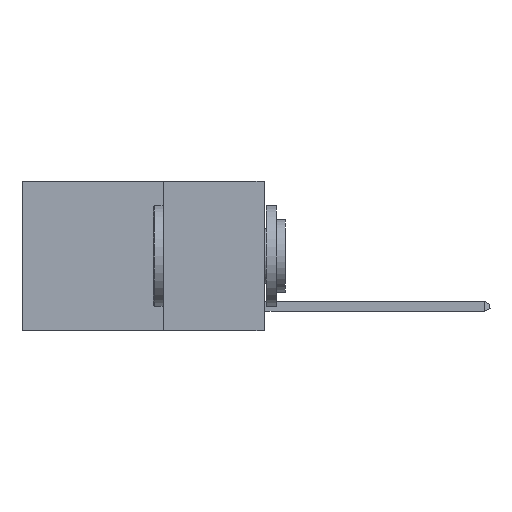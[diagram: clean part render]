
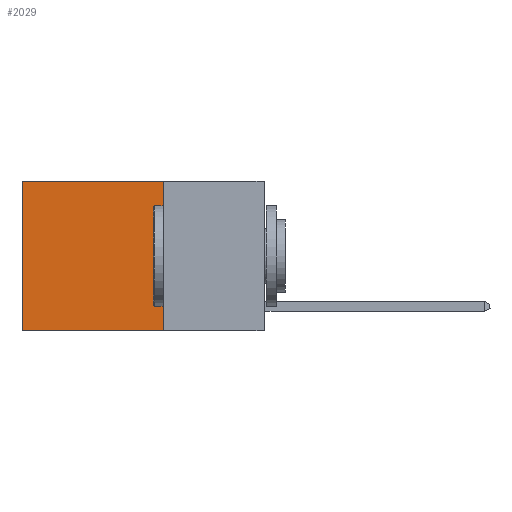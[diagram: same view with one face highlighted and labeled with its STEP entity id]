
A CAD part, left-side view. The second image highlights one B-rep face of the part: STEP entity #2029.
In plain terms, the highlighted planar face has unit normal (-1, 0, 0).
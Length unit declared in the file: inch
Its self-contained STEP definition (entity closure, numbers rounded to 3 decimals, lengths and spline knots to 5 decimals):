
#17 = CARTESIAN_POINT ( 'NONE',  ( 0.2625, 0.6, 0. ) ) ;
#695 = VECTOR ( 'NONE', #19083, 39.37008 ) ;
#1143 = LINE ( 'NONE', #16979, #18422 ) ;
#1632 = CARTESIAN_POINT ( 'NONE',  ( 0.2625, 0.6, 0. ) ) ;
#2029 = ADVANCED_FACE ( 'NONE', ( #10444 ), #10335, .F. ) ;
#2271 = AXIS2_PLACEMENT_3D ( 'NONE', #9075, #2316, #7178 ) ;
#2316 = DIRECTION ( 'NONE',  ( 1., 0., 0. ) ) ;
#5088 = CARTESIAN_POINT ( 'NONE',  ( 0.2625, 0.6, -0.37 ) ) ;
#5659 = ORIENTED_EDGE ( 'NONE', *, *, #8218, .F. ) ;
#6524 = LINE ( 'NONE', #16128, #695 ) ;
#6643 = EDGE_LOOP ( 'NONE', ( #17341, #8970, #5659, #12559 ) ) ;
#6662 = VERTEX_POINT ( 'NONE', #11390 ) ;
#7178 = DIRECTION ( 'NONE',  ( 0., 0., -1. ) ) ;
#7479 = VERTEX_POINT ( 'NONE', #5088 ) ;
#8218 = EDGE_CURVE ( 'NONE', #15869, #6662, #1143, .T. ) ;
#8365 = VECTOR ( 'NONE', #20331, 39.37008 ) ;
#8969 = DIRECTION ( 'NONE',  ( 0., 0., -1. ) ) ;
#8970 = ORIENTED_EDGE ( 'NONE', *, *, #12341, .F. ) ;
#9075 = CARTESIAN_POINT ( 'NONE',  ( 0.2625, 0.25, 0. ) ) ;
#10335 = PLANE ( 'NONE',  #2271 ) ;
#10444 = FACE_OUTER_BOUND ( 'NONE', #6643, .T. ) ;
#11390 = CARTESIAN_POINT ( 'NONE',  ( 0.2625, 0.25, -0.37 ) ) ;
#12341 = EDGE_CURVE ( 'NONE', #6662, #7479, #6524, .T. ) ;
#12559 = ORIENTED_EDGE ( 'NONE', *, *, #15182, .T. ) ;
#12908 = CARTESIAN_POINT ( 'NONE',  ( 0.2625, 0.25, 0. ) ) ;
#13112 = VERTEX_POINT ( 'NONE', #17 ) ;
#13894 = CARTESIAN_POINT ( 'NONE',  ( 0.2625, 0.25, 0. ) ) ;
#15182 = EDGE_CURVE ( 'NONE', #15869, #13112, #16646, .T. ) ;
#15769 = VECTOR ( 'NONE', #17975, 39.37008 ) ;
#15869 = VERTEX_POINT ( 'NONE', #12908 ) ;
#16128 = CARTESIAN_POINT ( 'NONE',  ( 0.2625, 0.25, -0.37 ) ) ;
#16503 = LINE ( 'NONE', #1632, #15769 ) ;
#16646 = LINE ( 'NONE', #13894, #8365 ) ;
#16979 = CARTESIAN_POINT ( 'NONE',  ( 0.2625, 0.25, 0. ) ) ;
#17222 = EDGE_CURVE ( 'NONE', #13112, #7479, #16503, .T. ) ;
#17341 = ORIENTED_EDGE ( 'NONE', *, *, #17222, .T. ) ;
#17975 = DIRECTION ( 'NONE',  ( 0., 0., -1. ) ) ;
#18422 = VECTOR ( 'NONE', #8969, 39.37008 ) ;
#19083 = DIRECTION ( 'NONE',  ( 0., 1., 0. ) ) ;
#20331 = DIRECTION ( 'NONE',  ( 0., 1., 0. ) ) ;
